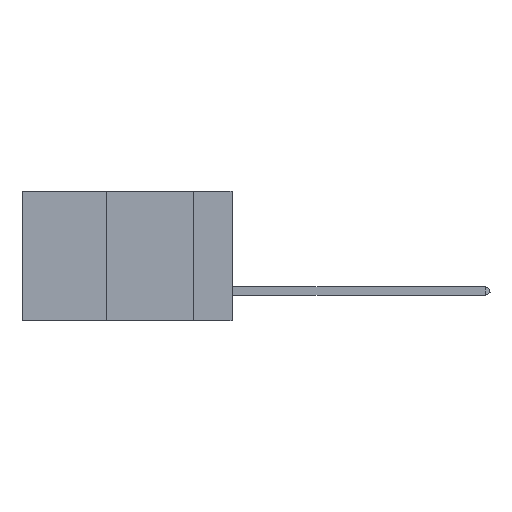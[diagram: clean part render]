
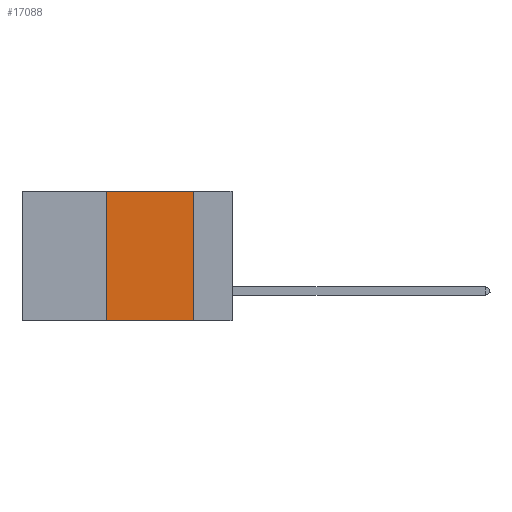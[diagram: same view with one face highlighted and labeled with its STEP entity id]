
A CAD part, left-side view. The second image highlights one B-rep face of the part: STEP entity #17088.
In plain terms, the highlighted planar face has unit normal (-1, 0, 0).
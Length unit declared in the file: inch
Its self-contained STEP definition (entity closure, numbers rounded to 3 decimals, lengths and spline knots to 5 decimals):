
#109 = CARTESIAN_POINT ( 'NONE',  ( 0., 0.11, 0. ) ) ;
#122 = VECTOR ( 'NONE', #9679, 39.37008 ) ;
#1378 = EDGE_CURVE ( 'NONE', #6553, #16835, #15671, .T. ) ;
#1664 = CARTESIAN_POINT ( 'NONE',  ( 0., 0.36, -0.37 ) ) ;
#1870 = ORIENTED_EDGE ( 'NONE', *, *, #11871, .T. ) ;
#2032 = DIRECTION ( 'NONE',  ( 1., 0., 0. ) ) ;
#2150 = VECTOR ( 'NONE', #23724, 39.37008 ) ;
#2588 = ORIENTED_EDGE ( 'NONE', *, *, #14216, .F. ) ;
#2779 = LINE ( 'NONE', #11384, #2150 ) ;
#3054 = EDGE_LOOP ( 'NONE', ( #26911, #2588, #7873, #1870 ) ) ;
#4159 = DIRECTION ( 'NONE',  ( 0., 0., -1. ) ) ;
#5425 = CARTESIAN_POINT ( 'NONE',  ( 0., 0.11, -0.37 ) ) ;
#5538 = DIRECTION ( 'NONE',  ( 0., 0., 1. ) ) ;
#6553 = VERTEX_POINT ( 'NONE', #109 ) ;
#7873 = ORIENTED_EDGE ( 'NONE', *, *, #13268, .F. ) ;
#8117 = DIRECTION ( 'NONE',  ( 0., -1., 0. ) ) ;
#9679 = DIRECTION ( 'NONE',  ( 0., 0., -1. ) ) ;
#10615 = VECTOR ( 'NONE', #8117, 39.37008 ) ;
#10717 = AXIS2_PLACEMENT_3D ( 'NONE', #17826, #2032, #4159 ) ;
#11384 = CARTESIAN_POINT ( 'NONE',  ( 0., 0.6, -0.37 ) ) ;
#11453 = CARTESIAN_POINT ( 'NONE',  ( 0., 0.36, 0. ) ) ;
#11871 = EDGE_CURVE ( 'NONE', #13530, #16835, #2779, .T. ) ;
#12213 = VERTEX_POINT ( 'NONE', #11453 ) ;
#13268 = EDGE_CURVE ( 'NONE', #13530, #12213, #25239, .T. ) ;
#13530 = VERTEX_POINT ( 'NONE', #1664 ) ;
#13842 = CARTESIAN_POINT ( 'NONE',  ( 0., 0.36, 0. ) ) ;
#14216 = EDGE_CURVE ( 'NONE', #12213, #6553, #14230, .T. ) ;
#14230 = LINE ( 'NONE', #23032, #10615 ) ;
#14397 = FACE_OUTER_BOUND ( 'NONE', #3054, .T. ) ;
#15671 = LINE ( 'NONE', #18124, #122 ) ;
#16835 = VERTEX_POINT ( 'NONE', #5425 ) ;
#17088 = ADVANCED_FACE ( 'NONE', ( #14397 ), #23215, .F. ) ;
#17826 = CARTESIAN_POINT ( 'NONE',  ( 0., 0.6, 0. ) ) ;
#18124 = CARTESIAN_POINT ( 'NONE',  ( 0., 0.11, 0. ) ) ;
#23032 = CARTESIAN_POINT ( 'NONE',  ( 0., 0.6, 0. ) ) ;
#23215 = PLANE ( 'NONE',  #10717 ) ;
#23724 = DIRECTION ( 'NONE',  ( 0., -1., 0. ) ) ;
#25239 = LINE ( 'NONE', #13842, #26893 ) ;
#26893 = VECTOR ( 'NONE', #5538, 39.37008 ) ;
#26911 = ORIENTED_EDGE ( 'NONE', *, *, #1378, .F. ) ;
